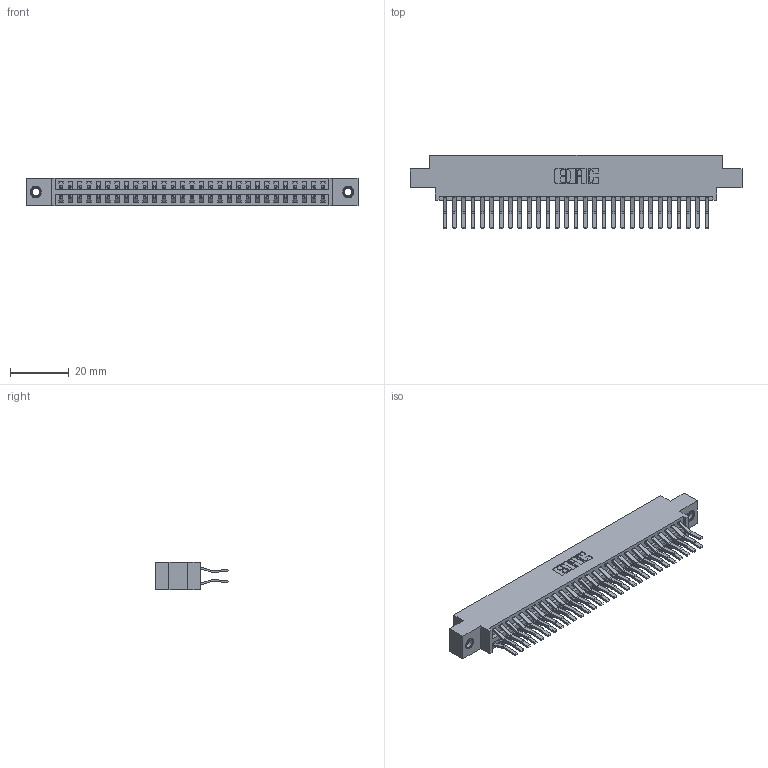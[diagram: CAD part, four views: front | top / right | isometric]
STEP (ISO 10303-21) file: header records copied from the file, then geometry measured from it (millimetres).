
FILE_DESCRIPTION (( 'STEP AP203' ), '1' );
FILE_NAME ('346-058-560-807.STEP', '2022-05-21T09:57:27', ( '' ), ( '' ), 'SwSTEP 2.0', 'SolidWorks 2020', '' );
FILE_SCHEMA (( 'CONFIG_CONTROL_DESIGN' ));
Length unit declared in the file: inch
Products named in the file (4): 346 Part_0.170 Offset - 0.156 Dia-TI; 345-250-001_345-250-005-103; 346-058-560-807; 345-292-001_560 Tail
Assembly tree (61 placements, depth 2):
  346-058-560-807
    346 Part_0.170 Offset - 0.156 Dia-TI
    345-292-001_560 Tail  x58
    345-250-001_345-250-005-103  x2
Bounding box: 112.65 x 24.78 x 9.4 mm (x, y, z)
Volume: 11095.7 mm3; surface area: 16275.2 mm2
Topology: 61 solids, 61 shells, 3318 faces, 9815 edges, 6458 vertices
Faces by surface type: plane 2142, cylinder 1160, cone 12, torus 4
Entity records: 22082 total; most frequent: CARTESIAN_POINT 3643, ORIENTED_EDGE 3570, DIRECTION 3291, EDGE_CURVE 1785, LINE 1513, VECTOR 1513, VERTEX_POINT 1184, AXIS2_PLACEMENT_3D 889
